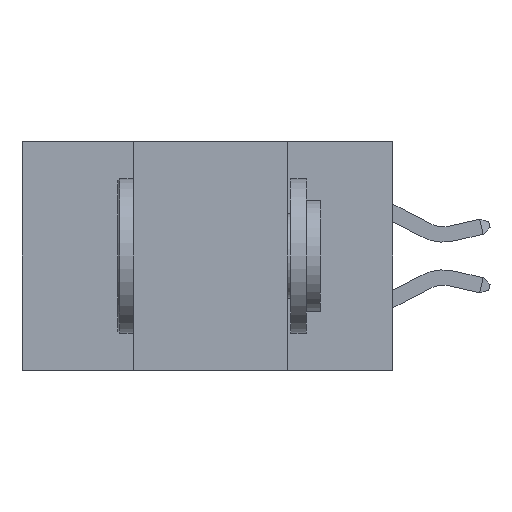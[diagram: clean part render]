
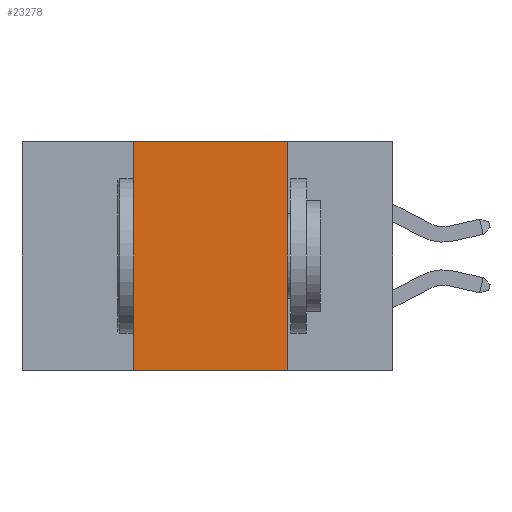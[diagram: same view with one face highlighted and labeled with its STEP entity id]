
A CAD part, left-side view. The second image highlights one B-rep face of the part: STEP entity #23278.
In plain terms, the highlighted planar face has unit normal (-1, 0, 0).
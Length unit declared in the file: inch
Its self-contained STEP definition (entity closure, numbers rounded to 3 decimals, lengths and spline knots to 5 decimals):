
#67 = VECTOR ( 'NONE', #21542, 39.37008 ) ;
#555 = CARTESIAN_POINT ( 'NONE',  ( 0., 0.42, 0. ) ) ;
#642 = DIRECTION ( 'NONE',  ( 0., 0., 1. ) ) ;
#1863 = ORIENTED_EDGE ( 'NONE', *, *, #26170, .F. ) ;
#2677 = VECTOR ( 'NONE', #20485, 39.37008 ) ;
#3439 = CARTESIAN_POINT ( 'NONE',  ( 0., 0.6, 0. ) ) ;
#6251 = DIRECTION ( 'NONE',  ( 0., 0., -1. ) ) ;
#6400 = FACE_OUTER_BOUND ( 'NONE', #20943, .T. ) ;
#8691 = CARTESIAN_POINT ( 'NONE',  ( 0., 0.42, -0.37 ) ) ;
#9473 = CARTESIAN_POINT ( 'NONE',  ( 0., 0.6, -0.37 ) ) ;
#10099 = LINE ( 'NONE', #9473, #2677 ) ;
#10469 = CARTESIAN_POINT ( 'NONE',  ( 0., 0.17, 0. ) ) ;
#13519 = VECTOR ( 'NONE', #29890, 39.37008 ) ;
#13753 = CARTESIAN_POINT ( 'NONE',  ( 0., 0.17, 0. ) ) ;
#13866 = EDGE_CURVE ( 'NONE', #17858, #24624, #10099, .T. ) ;
#16685 = VERTEX_POINT ( 'NONE', #555 ) ;
#17203 = PLANE ( 'NONE',  #19026 ) ;
#17345 = CARTESIAN_POINT ( 'NONE',  ( 0., 0.17, -0.37 ) ) ;
#17858 = VERTEX_POINT ( 'NONE', #8691 ) ;
#19026 = AXIS2_PLACEMENT_3D ( 'NONE', #3439, #22670, #6251 ) ;
#19125 = LINE ( 'NONE', #33313, #19989 ) ;
#19989 = VECTOR ( 'NONE', #642, 39.37008 ) ;
#20485 = DIRECTION ( 'NONE',  ( 0., -1., 0. ) ) ;
#20943 = EDGE_LOOP ( 'NONE', ( #32134, #23008, #1863, #28840 ) ) ;
#21542 = DIRECTION ( 'NONE',  ( 0., -1., 0. ) ) ;
#22670 = DIRECTION ( 'NONE',  ( 1., 0., 0. ) ) ;
#23008 = ORIENTED_EDGE ( 'NONE', *, *, #25906, .F. ) ;
#23278 = ADVANCED_FACE ( 'NONE', ( #6400 ), #17203, .F. ) ;
#24624 = VERTEX_POINT ( 'NONE', #17345 ) ;
#25906 = EDGE_CURVE ( 'NONE', #16685, #34666, #28392, .T. ) ;
#26170 = EDGE_CURVE ( 'NONE', #17858, #16685, #19125, .T. ) ;
#26567 = EDGE_CURVE ( 'NONE', #34666, #24624, #34978, .T. ) ;
#28392 = LINE ( 'NONE', #34828, #67 ) ;
#28840 = ORIENTED_EDGE ( 'NONE', *, *, #13866, .T. ) ;
#29890 = DIRECTION ( 'NONE',  ( 0., 0., -1. ) ) ;
#32134 = ORIENTED_EDGE ( 'NONE', *, *, #26567, .F. ) ;
#33313 = CARTESIAN_POINT ( 'NONE',  ( 0., 0.42, 0. ) ) ;
#34666 = VERTEX_POINT ( 'NONE', #10469 ) ;
#34828 = CARTESIAN_POINT ( 'NONE',  ( 0., 0.6, 0. ) ) ;
#34978 = LINE ( 'NONE', #13753, #13519 ) ;
